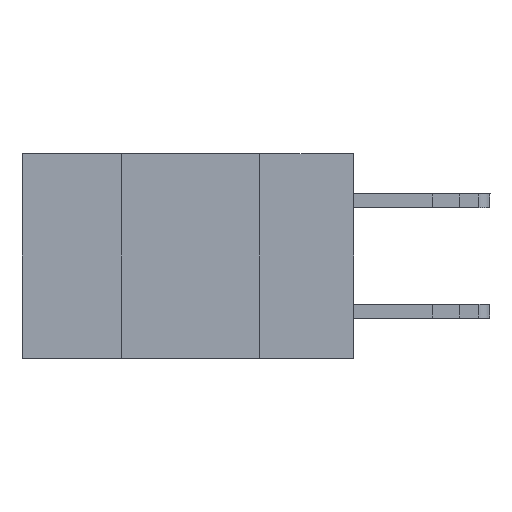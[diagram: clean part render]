
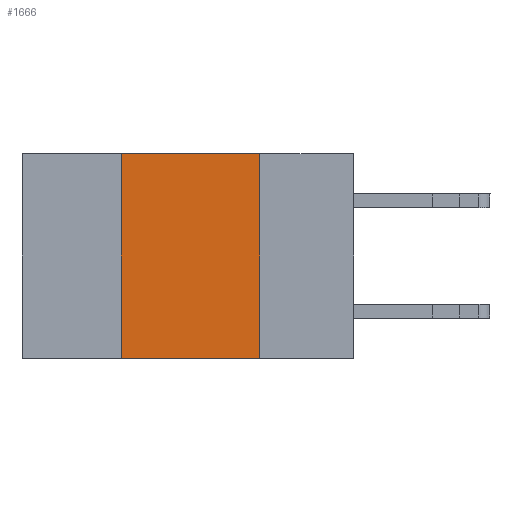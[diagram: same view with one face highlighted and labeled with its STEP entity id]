
A CAD part, left-side view. The second image highlights one B-rep face of the part: STEP entity #1666.
In plain terms, the highlighted planar face has unit normal (-1, 0, 0).
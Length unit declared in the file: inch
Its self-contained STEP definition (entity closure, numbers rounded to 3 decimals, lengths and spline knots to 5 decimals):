
#934 = LINE ( 'NONE', #3109, #17031 ) ;
#1015 = FACE_OUTER_BOUND ( 'NONE', #12436, .T. ) ;
#1264 = DIRECTION ( 'NONE',  ( 0., -1., 0. ) ) ;
#1666 = ADVANCED_FACE ( 'NONE', ( #1015 ), #7927, .F. ) ;
#1858 = CARTESIAN_POINT ( 'NONE',  ( 0., 0.17, -0.37 ) ) ;
#2203 = VERTEX_POINT ( 'NONE', #8660 ) ;
#2241 = ORIENTED_EDGE ( 'NONE', *, *, #13422, .F. ) ;
#3109 = CARTESIAN_POINT ( 'NONE',  ( 0., 0.6, 0. ) ) ;
#3529 = VECTOR ( 'NONE', #19212, 39.37008 ) ;
#4400 = ORIENTED_EDGE ( 'NONE', *, *, #14241, .F. ) ;
#5422 = VERTEX_POINT ( 'NONE', #1858 ) ;
#5844 = ORIENTED_EDGE ( 'NONE', *, *, #14473, .F. ) ;
#6950 = CARTESIAN_POINT ( 'NONE',  ( 0., 0.42, 0. ) ) ;
#7128 = CARTESIAN_POINT ( 'NONE',  ( 0., 0.42, -0.37 ) ) ;
#7927 = PLANE ( 'NONE',  #14003 ) ;
#8132 = CARTESIAN_POINT ( 'NONE',  ( 0., 0.42, 0. ) ) ;
#8267 = VERTEX_POINT ( 'NONE', #7128 ) ;
#8440 = CARTESIAN_POINT ( 'NONE',  ( 0., 0.17, 0. ) ) ;
#8660 = CARTESIAN_POINT ( 'NONE',  ( 0., 0.17, 0. ) ) ;
#9148 = DIRECTION ( 'NONE',  ( 1., 0., 0. ) ) ;
#9204 = DIRECTION ( 'NONE',  ( 0., 0., -1. ) ) ;
#9316 = CARTESIAN_POINT ( 'NONE',  ( 0., 0.6, 0. ) ) ;
#9684 = VERTEX_POINT ( 'NONE', #8132 ) ;
#9693 = ORIENTED_EDGE ( 'NONE', *, *, #17531, .T. ) ;
#10558 = LINE ( 'NONE', #19281, #16829 ) ;
#12016 = LINE ( 'NONE', #6950, #15135 ) ;
#12436 = EDGE_LOOP ( 'NONE', ( #4400, #5844, #2241, #9693 ) ) ;
#12712 = LINE ( 'NONE', #8440, #3529 ) ;
#13422 = EDGE_CURVE ( 'NONE', #8267, #9684, #12016, .T. ) ;
#14003 = AXIS2_PLACEMENT_3D ( 'NONE', #9316, #9148, #9204 ) ;
#14241 = EDGE_CURVE ( 'NONE', #2203, #5422, #12712, .T. ) ;
#14473 = EDGE_CURVE ( 'NONE', #9684, #2203, #934, .T. ) ;
#15135 = VECTOR ( 'NONE', #17570, 39.37008 ) ;
#15426 = DIRECTION ( 'NONE',  ( 0., -1., 0. ) ) ;
#16829 = VECTOR ( 'NONE', #1264, 39.37008 ) ;
#17031 = VECTOR ( 'NONE', #15426, 39.37008 ) ;
#17531 = EDGE_CURVE ( 'NONE', #8267, #5422, #10558, .T. ) ;
#17570 = DIRECTION ( 'NONE',  ( 0., 0., 1. ) ) ;
#19212 = DIRECTION ( 'NONE',  ( 0., 0., -1. ) ) ;
#19281 = CARTESIAN_POINT ( 'NONE',  ( 0., 0.6, -0.37 ) ) ;
